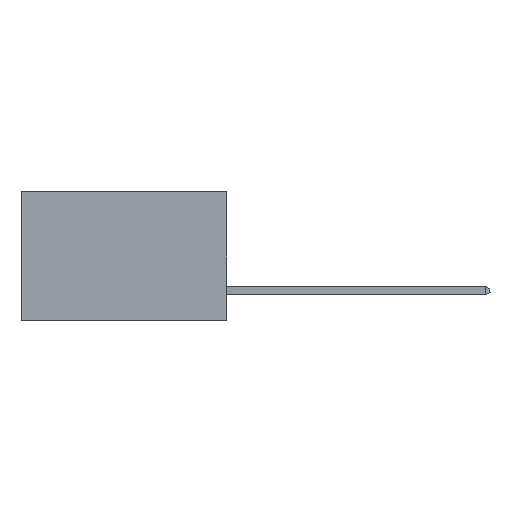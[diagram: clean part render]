
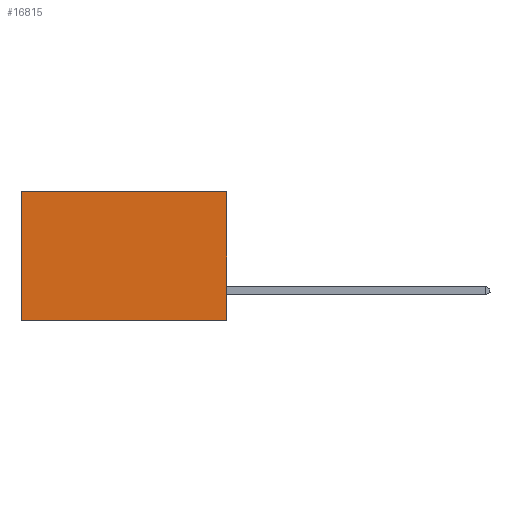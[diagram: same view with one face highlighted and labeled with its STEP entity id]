
A CAD part, left-side view. The second image highlights one B-rep face of the part: STEP entity #16815.
In plain terms, the highlighted planar face has unit normal (-1, 0, 0).
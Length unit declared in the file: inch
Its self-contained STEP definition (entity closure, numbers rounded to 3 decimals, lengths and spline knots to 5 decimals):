
#256 = CARTESIAN_POINT ( 'NONE',  ( 0.277, 0.59, 0. ) ) ;
#474 = DIRECTION ( 'NONE',  ( 0., 1., 0. ) ) ;
#762 = CARTESIAN_POINT ( 'NONE',  ( 0.277, 0., 0. ) ) ;
#918 = ORIENTED_EDGE ( 'NONE', *, *, #14206, .T. ) ;
#1138 = VECTOR ( 'NONE', #3270, 39.37008 ) ;
#1490 = CARTESIAN_POINT ( 'NONE',  ( 0.277, 0., -0.37 ) ) ;
#1806 = EDGE_LOOP ( 'NONE', ( #918, #9098, #10281, #2557 ) ) ;
#2557 = ORIENTED_EDGE ( 'NONE', *, *, #19371, .T. ) ;
#3270 = DIRECTION ( 'NONE',  ( 0., 0., -1. ) ) ;
#4021 = CARTESIAN_POINT ( 'NONE',  ( 0.277, 0., -0.37 ) ) ;
#4229 = DIRECTION ( 'NONE',  ( 0., 1., 0. ) ) ;
#4437 = LINE ( 'NONE', #762, #4968 ) ;
#4968 = VECTOR ( 'NONE', #4229, 39.37008 ) ;
#5745 = DIRECTION ( 'NONE',  ( 1., 0., 0. ) ) ;
#6325 = LINE ( 'NONE', #1490, #1138 ) ;
#7785 = CARTESIAN_POINT ( 'NONE',  ( 0.277, 0., -0.37 ) ) ;
#8657 = EDGE_CURVE ( 'NONE', #12503, #21356, #6325, .T. ) ;
#8981 = LINE ( 'NONE', #8990, #22184 ) ;
#8990 = CARTESIAN_POINT ( 'NONE',  ( 0.277, 0.59, -0.37 ) ) ;
#9098 = ORIENTED_EDGE ( 'NONE', *, *, #16800, .F. ) ;
#10260 = VECTOR ( 'NONE', #474, 39.37008 ) ;
#10281 = ORIENTED_EDGE ( 'NONE', *, *, #8657, .F. ) ;
#12503 = VERTEX_POINT ( 'NONE', #22342 ) ;
#12648 = VERTEX_POINT ( 'NONE', #256 ) ;
#14206 = EDGE_CURVE ( 'NONE', #12648, #21385, #8981, .T. ) ;
#14868 = CARTESIAN_POINT ( 'NONE',  ( 0.277, 0.59, -0.37 ) ) ;
#14879 = FACE_OUTER_BOUND ( 'NONE', #1806, .T. ) ;
#16145 = PLANE ( 'NONE',  #21213 ) ;
#16800 = EDGE_CURVE ( 'NONE', #21356, #21385, #19951, .T. ) ;
#16815 = ADVANCED_FACE ( 'NONE', ( #14879 ), #16145, .F. ) ;
#17668 = DIRECTION ( 'NONE',  ( 0., 0., -1. ) ) ;
#17843 = DIRECTION ( 'NONE',  ( 0., 0., -1. ) ) ;
#19371 = EDGE_CURVE ( 'NONE', #12503, #12648, #4437, .T. ) ;
#19951 = LINE ( 'NONE', #21221, #10260 ) ;
#21213 = AXIS2_PLACEMENT_3D ( 'NONE', #4021, #5745, #17843 ) ;
#21221 = CARTESIAN_POINT ( 'NONE',  ( 0.277, 0., -0.37 ) ) ;
#21356 = VERTEX_POINT ( 'NONE', #7785 ) ;
#21385 = VERTEX_POINT ( 'NONE', #14868 ) ;
#22184 = VECTOR ( 'NONE', #17668, 39.37008 ) ;
#22342 = CARTESIAN_POINT ( 'NONE',  ( 0.277, 0., 0. ) ) ;
